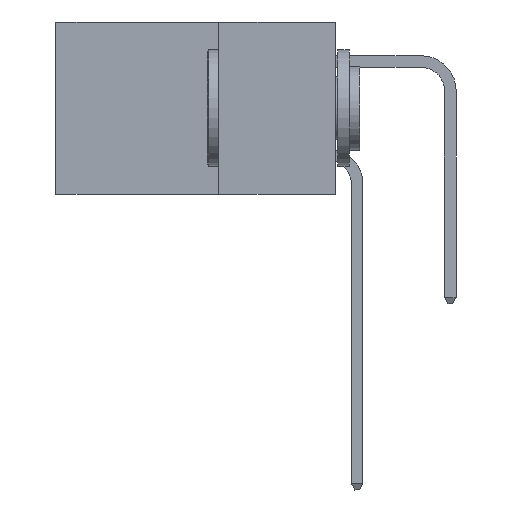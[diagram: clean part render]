
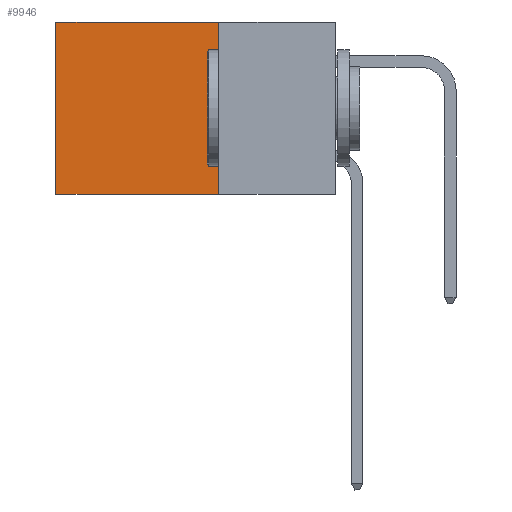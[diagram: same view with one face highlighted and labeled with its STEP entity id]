
A CAD part, left-side view. The second image highlights one B-rep face of the part: STEP entity #9946.
In plain terms, the highlighted planar face has unit normal (-1, 0, 0).
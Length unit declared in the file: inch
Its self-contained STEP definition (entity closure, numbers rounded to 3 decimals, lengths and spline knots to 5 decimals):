
#212 = PLANE ( 'NONE',  #11352 ) ;
#1554 = VECTOR ( 'NONE', #23250, 39.37008 ) ;
#2354 = ORIENTED_EDGE ( 'NONE', *, *, #4311, .F. ) ;
#2513 = DIRECTION ( 'NONE',  ( 0., 0., -1. ) ) ;
#3735 = EDGE_CURVE ( 'NONE', #20028, #16409, #4087, .T. ) ;
#3961 = VECTOR ( 'NONE', #5349, 39.37008 ) ;
#4087 = LINE ( 'NONE', #23520, #13739 ) ;
#4178 = EDGE_LOOP ( 'NONE', ( #21954, #2354, #23144, #12846 ) ) ;
#4311 = EDGE_CURVE ( 'NONE', #6459, #16409, #6822, .T. ) ;
#5349 = DIRECTION ( 'NONE',  ( 0., 1., 0. ) ) ;
#6459 = VERTEX_POINT ( 'NONE', #12028 ) ;
#6792 = EDGE_CURVE ( 'NONE', #10073, #20028, #24256, .T. ) ;
#6822 = LINE ( 'NONE', #11925, #1554 ) ;
#8198 = DIRECTION ( 'NONE',  ( 0., 0., -1. ) ) ;
#8207 = CARTESIAN_POINT ( 'NONE',  ( 0.2875, 0.25, 0. ) ) ;
#9946 = ADVANCED_FACE ( 'NONE', ( #23497 ), #212, .F. ) ;
#10073 = VERTEX_POINT ( 'NONE', #23931 ) ;
#10126 = DIRECTION ( 'NONE',  ( 0., 0., -1. ) ) ;
#11352 = AXIS2_PLACEMENT_3D ( 'NONE', #8207, #21488, #10126 ) ;
#11588 = EDGE_CURVE ( 'NONE', #10073, #6459, #12461, .T. ) ;
#11925 = CARTESIAN_POINT ( 'NONE',  ( 0.2875, 0.25, -0.37 ) ) ;
#12028 = CARTESIAN_POINT ( 'NONE',  ( 0.2875, 0.25, -0.37 ) ) ;
#12461 = LINE ( 'NONE', #19669, #16895 ) ;
#12846 = ORIENTED_EDGE ( 'NONE', *, *, #6792, .T. ) ;
#13739 = VECTOR ( 'NONE', #2513, 39.37008 ) ;
#15003 = CARTESIAN_POINT ( 'NONE',  ( 0.2875, 0.6, -0.37 ) ) ;
#16409 = VERTEX_POINT ( 'NONE', #15003 ) ;
#16895 = VECTOR ( 'NONE', #8198, 39.37008 ) ;
#19669 = CARTESIAN_POINT ( 'NONE',  ( 0.2875, 0.25, 0. ) ) ;
#20028 = VERTEX_POINT ( 'NONE', #23132 ) ;
#20661 = CARTESIAN_POINT ( 'NONE',  ( 0.2875, 0.25, 0. ) ) ;
#21488 = DIRECTION ( 'NONE',  ( 1., 0., 0. ) ) ;
#21954 = ORIENTED_EDGE ( 'NONE', *, *, #3735, .T. ) ;
#23132 = CARTESIAN_POINT ( 'NONE',  ( 0.2875, 0.6, 0. ) ) ;
#23144 = ORIENTED_EDGE ( 'NONE', *, *, #11588, .F. ) ;
#23250 = DIRECTION ( 'NONE',  ( 0., 1., 0. ) ) ;
#23497 = FACE_OUTER_BOUND ( 'NONE', #4178, .T. ) ;
#23520 = CARTESIAN_POINT ( 'NONE',  ( 0.2875, 0.6, 0. ) ) ;
#23931 = CARTESIAN_POINT ( 'NONE',  ( 0.2875, 0.25, 0. ) ) ;
#24256 = LINE ( 'NONE', #20661, #3961 ) ;
